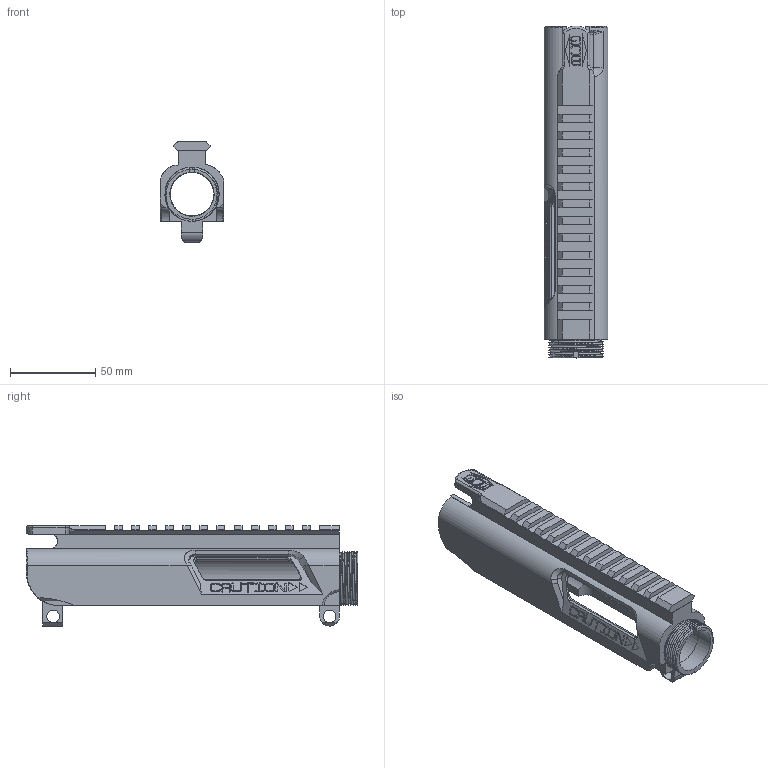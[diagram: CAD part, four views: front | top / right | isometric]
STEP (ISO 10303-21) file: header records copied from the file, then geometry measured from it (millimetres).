
FILE_DESCRIPTION(/* description */ (''),/* implementation_level */ '2;1');
FILE_NAME(/* name */ 'SG22 Upper Release.step',/* time_stamp */ '2021-03-18T08:52:52-06:00',/* author */ (''),/* organization */ (''),/* preprocessor_version */ 'ST-DEVELOPER v18.1',/* originating_system */ 'Autodesk Translation Framework v9.10.0.1330',/* authorisation */ '');
FILE_SCHEMA (('AUTOMOTIVE_DESIGN { 1 0 10303 214 3 1 1 }'));
Length unit declared in the file: millimetre
Products named in the file (1): Brace V2
Bounding box: 37.37 x 194.4 x 59 mm (x, y, z)
Volume: 111829.5 mm3; surface area: 52456.8 mm2
Topology: 1 solids, 1 shells, 682 faces, 1949 edges, 1282 vertices
Faces by surface type: plane 396, bspline 143, cylinder 87, cone 50, torus 6
Full cylindrical faces by diameter (mm): 7.35 x1, 7.358 x1, 25.546 x1, 25.927 x1, 29.782 x1, 31.7 x4
Entity records: 25076 total; most frequent: CARTESIAN_POINT 8711, ORIENTED_EDGE 3890, DIRECTION 2780, EDGE_CURVE 1945, LINE 1296, VECTOR 1296, VERTEX_POINT 1282, AXIS2_PLACEMENT_3D 742
